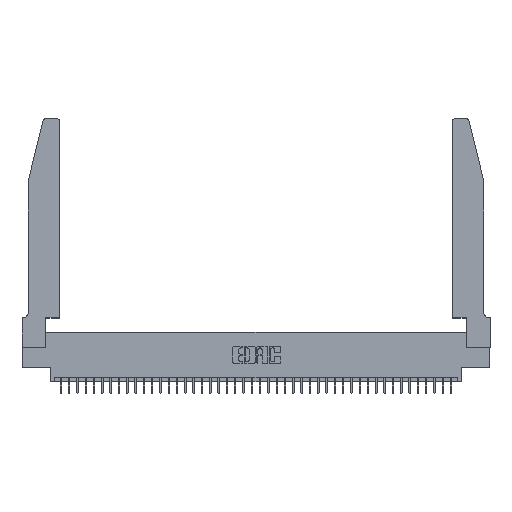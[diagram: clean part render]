
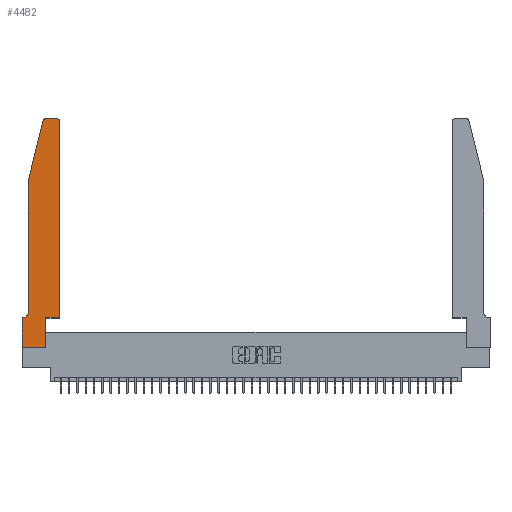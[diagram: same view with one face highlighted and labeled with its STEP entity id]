
A CAD part, top view. The second image highlights one B-rep face of the part: STEP entity #4482.
In plain terms, the highlighted planar face has unit normal (0, 0, 1).
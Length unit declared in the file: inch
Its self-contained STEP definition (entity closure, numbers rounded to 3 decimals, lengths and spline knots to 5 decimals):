
#18 = EDGE_LOOP ( 'NONE', ( #38442, #1337, #5692, #13285, #34389, #31790, #23227, #20343, #32638, #28873, #26666, #8789 ) ) ;
#221 = VECTOR ( 'NONE', #30239, 39.37008 ) ;
#878 = VECTOR ( 'NONE', #28969, 39.37008 ) ;
#1337 = ORIENTED_EDGE ( 'NONE', *, *, #16475, .T. ) ;
#1354 = DIRECTION ( 'NONE',  ( 0., 0., 1. ) ) ;
#1383 = VERTEX_POINT ( 'NONE', #11430 ) ;
#1630 = EDGE_CURVE ( 'NONE', #14585, #3748, #7570, .T. ) ;
#2957 = DIRECTION ( 'NONE',  ( 0., 1., 0. ) ) ;
#2992 = CARTESIAN_POINT ( 'NONE',  ( 0.0755, 2., 0.37 ) ) ;
#3691 = FACE_OUTER_BOUND ( 'NONE', #18, .T. ) ;
#3748 = VERTEX_POINT ( 'NONE', #21010 ) ;
#3899 = CARTESIAN_POINT ( 'NONE',  ( 0.4205, 2.72, 0.37 ) ) ;
#4018 = CARTESIAN_POINT ( 'NONE',  ( 0.2865, 0.35, 0.37 ) ) ;
#4482 = ADVANCED_FACE ( 'NONE', ( #3691 ), #39264, .T. ) ;
#4606 = LINE ( 'NONE', #30674, #221 ) ;
#5190 = EDGE_CURVE ( 'NONE', #1383, #25726, #37892, .T. ) ;
#5692 = ORIENTED_EDGE ( 'NONE', *, *, #25887, .T. ) ;
#5786 = CARTESIAN_POINT ( 'NONE',  ( 0.284, 2.72, 0.37 ) ) ;
#7570 = LINE ( 'NONE', #23447, #30546 ) ;
#8289 = AXIS2_PLACEMENT_3D ( 'NONE', #23173, #17239, #17450 ) ;
#8293 = CARTESIAN_POINT ( 'NONE',  ( 0.2605, 2.75, 0.37 ) ) ;
#8527 = DIRECTION ( 'NONE',  ( -1., 0., 0. ) ) ;
#8789 = ORIENTED_EDGE ( 'NONE', *, *, #22369, .T. ) ;
#9064 = CARTESIAN_POINT ( 'NONE',  ( 0.2865, 0., 0.37 ) ) ;
#9501 = EDGE_CURVE ( 'NONE', #10031, #1383, #14155, .T. ) ;
#9870 = EDGE_CURVE ( 'NONE', #21846, #12658, #30440, .T. ) ;
#10031 = VERTEX_POINT ( 'NONE', #9064 ) ;
#10557 = VERTEX_POINT ( 'NONE', #17366 ) ;
#11084 = EDGE_CURVE ( 'NONE', #3748, #10557, #4606, .T. ) ;
#11231 = DIRECTION ( 'NONE',  ( 0., 1., 0. ) ) ;
#11269 = AXIS2_PLACEMENT_3D ( 'NONE', #5786, #27582, #25043 ) ;
#11430 = CARTESIAN_POINT ( 'NONE',  ( 0.2865, 0.35, 0.37 ) ) ;
#12658 = VERTEX_POINT ( 'NONE', #35923 ) ;
#13285 = ORIENTED_EDGE ( 'NONE', *, *, #9870, .T. ) ;
#13399 = VECTOR ( 'NONE', #29482, 39.37008 ) ;
#13464 = VERTEX_POINT ( 'NONE', #40555 ) ;
#14155 = LINE ( 'NONE', #4018, #37392 ) ;
#14176 = CIRCLE ( 'NONE', #18927, 0.03 ) ;
#14202 = LINE ( 'NONE', #29918, #13399 ) ;
#14585 = VERTEX_POINT ( 'NONE', #39923 ) ;
#16475 = EDGE_CURVE ( 'NONE', #17274, #13464, #18701, .T. ) ;
#17239 = DIRECTION ( 'NONE',  ( 0., 0., 1. ) ) ;
#17250 = DIRECTION ( 'NONE',  ( 1., 0., 0. ) ) ;
#17274 = VERTEX_POINT ( 'NONE', #21963 ) ;
#17308 = DIRECTION ( 'NONE',  ( -1., 0., 0. ) ) ;
#17309 = CARTESIAN_POINT ( 'NONE',  ( 0.0755, 2., 0.37 ) ) ;
#17366 = CARTESIAN_POINT ( 'NONE',  ( 0., 0., 0.37 ) ) ;
#17450 = DIRECTION ( 'NONE',  ( 1., 0., 0. ) ) ;
#18701 = CIRCLE ( 'NONE', #11269, 0.03 ) ;
#18927 = AXIS2_PLACEMENT_3D ( 'NONE', #3899, #1354, #17250 ) ;
#18993 = VECTOR ( 'NONE', #28940, 39.37008 ) ;
#19436 = CARTESIAN_POINT ( 'NONE',  ( 0.4505, 0.35, 0.37 ) ) ;
#20343 = ORIENTED_EDGE ( 'NONE', *, *, #39719, .T. ) ;
#20563 = CARTESIAN_POINT ( 'NONE',  ( 0.4205, 2.75, 0.37 ) ) ;
#20770 = AXIS2_PLACEMENT_3D ( 'NONE', #24391, #40934, #8527 ) ;
#21010 = CARTESIAN_POINT ( 'NONE',  ( 0., 0.35, 0.37 ) ) ;
#21846 = VERTEX_POINT ( 'NONE', #2992 ) ;
#21963 = CARTESIAN_POINT ( 'NONE',  ( 0.284, 2.75, 0.37 ) ) ;
#22369 = EDGE_CURVE ( 'NONE', #27008, #33975, #14176, .T. ) ;
#22926 = CARTESIAN_POINT ( 'NONE',  ( 0.4505, 2.72, 0.37 ) ) ;
#23173 = CARTESIAN_POINT ( 'NONE',  ( 0., 0.35, 0.37 ) ) ;
#23227 = ORIENTED_EDGE ( 'NONE', *, *, #11084, .T. ) ;
#23243 = DIRECTION ( 'NONE',  ( 0., -1., 0. ) ) ;
#23447 = CARTESIAN_POINT ( 'NONE',  ( 0.0755, 0.35, 0.37 ) ) ;
#23472 = CIRCLE ( 'NONE', #20770, 0.07 ) ;
#24264 = EDGE_CURVE ( 'NONE', #12658, #14585, #23472, .T. ) ;
#24391 = CARTESIAN_POINT ( 'NONE',  ( 0.0055, 0.42, 0.37 ) ) ;
#24939 = EDGE_CURVE ( 'NONE', #25726, #27008, #38114, .T. ) ;
#25043 = DIRECTION ( 'NONE',  ( 1., 0., 0. ) ) ;
#25726 = VERTEX_POINT ( 'NONE', #31647 ) ;
#25887 = EDGE_CURVE ( 'NONE', #13464, #21846, #14202, .T. ) ;
#26666 = ORIENTED_EDGE ( 'NONE', *, *, #24939, .T. ) ;
#27008 = VERTEX_POINT ( 'NONE', #22926 ) ;
#27582 = DIRECTION ( 'NONE',  ( 0., 0., 1. ) ) ;
#28873 = ORIENTED_EDGE ( 'NONE', *, *, #5190, .T. ) ;
#28924 = VECTOR ( 'NONE', #2957, 39.37008 ) ;
#28940 = DIRECTION ( 'NONE',  ( 1., 0., 0. ) ) ;
#28969 = DIRECTION ( 'NONE',  ( 1., 0., 0. ) ) ;
#29482 = DIRECTION ( 'NONE',  ( -0.239, -0.971, 0. ) ) ;
#29918 = CARTESIAN_POINT ( 'NONE',  ( 0.0755, 2., 0.37 ) ) ;
#30239 = DIRECTION ( 'NONE',  ( 0., -1., 0. ) ) ;
#30440 = LINE ( 'NONE', #17309, #31285 ) ;
#30546 = VECTOR ( 'NONE', #17308, 39.37008 ) ;
#30674 = CARTESIAN_POINT ( 'NONE',  ( 0., 0., 0.37 ) ) ;
#31285 = VECTOR ( 'NONE', #23243, 39.37008 ) ;
#31647 = CARTESIAN_POINT ( 'NONE',  ( 0.4505, 0.35, 0.37 ) ) ;
#31790 = ORIENTED_EDGE ( 'NONE', *, *, #1630, .T. ) ;
#32162 = CARTESIAN_POINT ( 'NONE',  ( 0.4505, 0.35, 0.37 ) ) ;
#32638 = ORIENTED_EDGE ( 'NONE', *, *, #9501, .T. ) ;
#32746 = EDGE_CURVE ( 'NONE', #33975, #17274, #37102, .T. ) ;
#33975 = VERTEX_POINT ( 'NONE', #20563 ) ;
#34149 = DIRECTION ( 'NONE',  ( -1., 0., 0. ) ) ;
#34389 = ORIENTED_EDGE ( 'NONE', *, *, #24264, .T. ) ;
#35514 = LINE ( 'NONE', #41254, #18993 ) ;
#35923 = CARTESIAN_POINT ( 'NONE',  ( 0.0755, 0.42, 0.37 ) ) ;
#37102 = LINE ( 'NONE', #8293, #40106 ) ;
#37392 = VECTOR ( 'NONE', #11231, 39.37008 ) ;
#37892 = LINE ( 'NONE', #19436, #878 ) ;
#38114 = LINE ( 'NONE', #32162, #28924 ) ;
#38442 = ORIENTED_EDGE ( 'NONE', *, *, #32746, .T. ) ;
#39264 = PLANE ( 'NONE',  #8289 ) ;
#39719 = EDGE_CURVE ( 'NONE', #10557, #10031, #35514, .T. ) ;
#39923 = CARTESIAN_POINT ( 'NONE',  ( 0.0055, 0.35, 0.37 ) ) ;
#40106 = VECTOR ( 'NONE', #34149, 39.37008 ) ;
#40555 = CARTESIAN_POINT ( 'NONE',  ( 0.25487, 2.72718, 0.37 ) ) ;
#40934 = DIRECTION ( 'NONE',  ( 0., 0., -1. ) ) ;
#41254 = CARTESIAN_POINT ( 'NONE',  ( 0., 0., 0.37 ) ) ;
